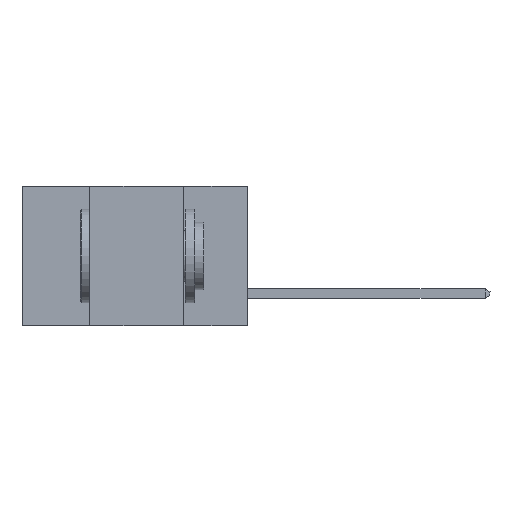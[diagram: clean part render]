
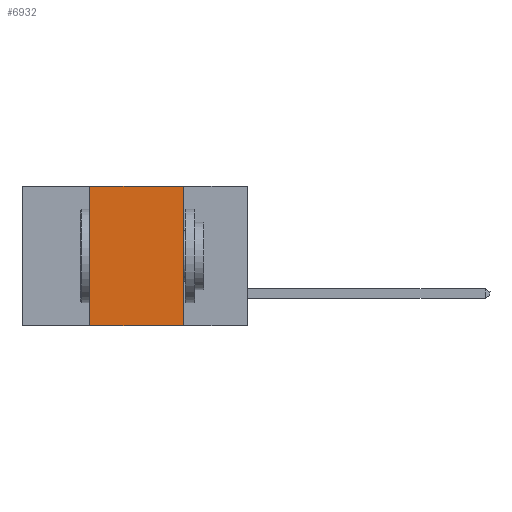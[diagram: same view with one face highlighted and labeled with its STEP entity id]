
A CAD part, left-side view. The second image highlights one B-rep face of the part: STEP entity #6932.
In plain terms, the highlighted planar face has unit normal (-1, 0, 0).
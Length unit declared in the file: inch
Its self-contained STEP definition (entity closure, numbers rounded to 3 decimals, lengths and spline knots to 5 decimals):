
#136 = AXIS2_PLACEMENT_3D ( 'NONE', #8891, #1158, #8165 ) ;
#386 = DIRECTION ( 'NONE',  ( 0., 0., 1. ) ) ;
#614 = VERTEX_POINT ( 'NONE', #8594 ) ;
#715 = CARTESIAN_POINT ( 'NONE',  ( 0., 0.17, -0.37 ) ) ;
#888 = EDGE_CURVE ( 'NONE', #1609, #614, #7568, .T. ) ;
#894 = CARTESIAN_POINT ( 'NONE',  ( 0., 0.17, 0. ) ) ;
#947 = DIRECTION ( 'NONE',  ( 0., -1., 0. ) ) ;
#1158 = DIRECTION ( 'NONE',  ( 1., 0., 0. ) ) ;
#1324 = EDGE_CURVE ( 'NONE', #1609, #8758, #8169, .T. ) ;
#1540 = CARTESIAN_POINT ( 'NONE',  ( 0., 0.42, -0.37 ) ) ;
#1609 = VERTEX_POINT ( 'NONE', #1540 ) ;
#1902 = DIRECTION ( 'NONE',  ( 0., -1., 0. ) ) ;
#1910 = ORIENTED_EDGE ( 'NONE', *, *, #888, .F. ) ;
#1919 = CARTESIAN_POINT ( 'NONE',  ( 0., 0.42, -0.37 ) ) ;
#2257 = EDGE_LOOP ( 'NONE', ( #4228, #8624, #1910, #4419 ) ) ;
#2299 = LINE ( 'NONE', #6000, #3862 ) ;
#2366 = EDGE_CURVE ( 'NONE', #5568, #8758, #4423, .T. ) ;
#2508 = EDGE_CURVE ( 'NONE', #614, #5568, #2299, .T. ) ;
#2762 = DIRECTION ( 'NONE',  ( 0., 0., -1. ) ) ;
#3862 = VECTOR ( 'NONE', #947, 39.37008 ) ;
#4129 = FACE_OUTER_BOUND ( 'NONE', #2257, .T. ) ;
#4228 = ORIENTED_EDGE ( 'NONE', *, *, #2366, .F. ) ;
#4419 = ORIENTED_EDGE ( 'NONE', *, *, #1324, .T. ) ;
#4423 = LINE ( 'NONE', #715, #8823 ) ;
#4585 = CARTESIAN_POINT ( 'NONE',  ( 0., 0.17, -0.37 ) ) ;
#5568 = VERTEX_POINT ( 'NONE', #894 ) ;
#6000 = CARTESIAN_POINT ( 'NONE',  ( 0., 0.6, 0. ) ) ;
#6096 = CARTESIAN_POINT ( 'NONE',  ( 0., 0.6, -0.37 ) ) ;
#6865 = PLANE ( 'NONE',  #136 ) ;
#6932 = ADVANCED_FACE ( 'NONE', ( #4129 ), #6865, .F. ) ;
#7138 = VECTOR ( 'NONE', #1902, 39.37008 ) ;
#7559 = VECTOR ( 'NONE', #386, 39.37008 ) ;
#7568 = LINE ( 'NONE', #1919, #7559 ) ;
#8165 = DIRECTION ( 'NONE',  ( 0., 0., -1. ) ) ;
#8169 = LINE ( 'NONE', #6096, #7138 ) ;
#8594 = CARTESIAN_POINT ( 'NONE',  ( 0., 0.42, 0. ) ) ;
#8624 = ORIENTED_EDGE ( 'NONE', *, *, #2508, .F. ) ;
#8758 = VERTEX_POINT ( 'NONE', #4585 ) ;
#8823 = VECTOR ( 'NONE', #2762, 39.37008 ) ;
#8891 = CARTESIAN_POINT ( 'NONE',  ( 0., 0.6, 0. ) ) ;
